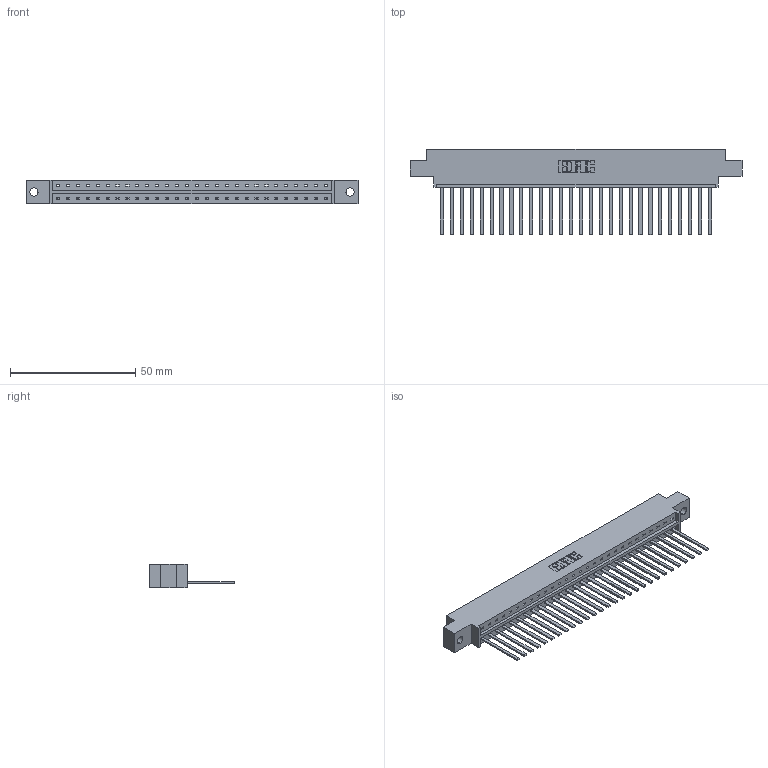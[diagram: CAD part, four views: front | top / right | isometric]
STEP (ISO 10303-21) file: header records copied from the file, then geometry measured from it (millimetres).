
FILE_DESCRIPTION (( 'STEP AP203' ), '1' );
FILE_NAME ('333-028-544-602.STEP', '2018-08-02T15:31:58', ( '' ), ( '' ), 'SwSTEP 2.0', 'SolidWorks 2016', '' );
FILE_SCHEMA (( 'CONFIG_CONTROL_DESIGN' ));
Length unit declared in the file: inch
Products named in the file (3): 333 Part_Offset - .128 Dia; 345-292-001_345-293-144; 333-028-544-602
Assembly tree (29 placements, depth 2):
  333-028-544-602
    333 Part_Offset - .128 Dia
    345-292-001_345-293-144  x28
Bounding box: 132.49 x 34.3 x 9.4 mm (x, y, z)
Volume: 13271.3 mm3; surface area: 15247.8 mm2
Topology: 29 solids, 29 shells, 1574 faces, 4747 edges, 3126 vertices
Faces by surface type: plane 1138, cylinder 436
Entity records: 18879 total; most frequent: CARTESIAN_POINT 3266, ORIENTED_EDGE 3230, DIRECTION 2779, EDGE_CURVE 1615, VECTOR 1491, LINE 1491, VERTEX_POINT 1074, AXIS2_PLACEMENT_3D 644
